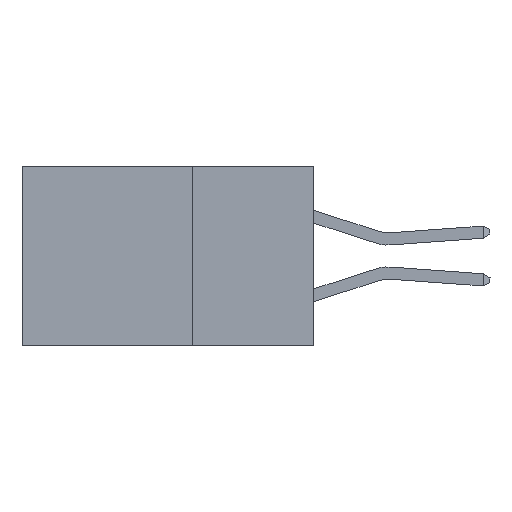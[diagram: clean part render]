
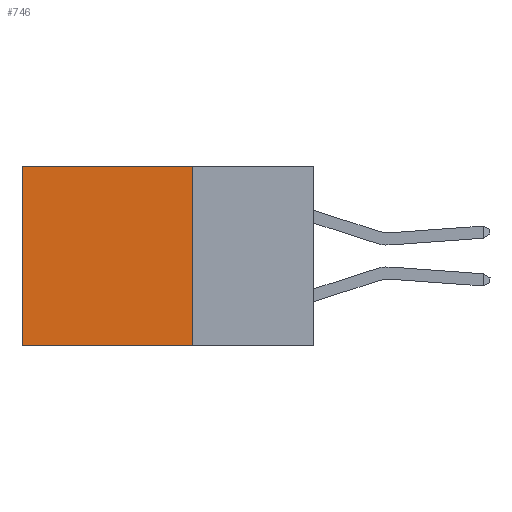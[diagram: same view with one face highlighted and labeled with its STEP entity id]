
A CAD part, left-side view. The second image highlights one B-rep face of the part: STEP entity #746.
In plain terms, the highlighted planar face has unit normal (-1, 0, 0).
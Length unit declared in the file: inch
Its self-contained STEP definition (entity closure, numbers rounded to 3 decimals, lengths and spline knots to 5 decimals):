
#235 = CARTESIAN_POINT ( 'NONE',  ( 0.2875, 0.25, -0.37 ) ) ;
#746 = ADVANCED_FACE ( 'NONE', ( #23379 ), #26019, .F. ) ;
#1162 = CARTESIAN_POINT ( 'NONE',  ( 0.2875, 0.25, 0. ) ) ;
#1590 = VERTEX_POINT ( 'NONE', #28238 ) ;
#2686 = DIRECTION ( 'NONE',  ( 0., 0., -1. ) ) ;
#2745 = CARTESIAN_POINT ( 'NONE',  ( 0.2875, 0.25, 0. ) ) ;
#2875 = DIRECTION ( 'NONE',  ( 0., 1., 0. ) ) ;
#3128 = CARTESIAN_POINT ( 'NONE',  ( 0.2875, 0.6, -0.37 ) ) ;
#3376 = DIRECTION ( 'NONE',  ( 1., 0., 0. ) ) ;
#5682 = EDGE_CURVE ( 'NONE', #7525, #10924, #10752, .T. ) ;
#6465 = EDGE_CURVE ( 'NONE', #19466, #7525, #8320, .T. ) ;
#6934 = ORIENTED_EDGE ( 'NONE', *, *, #10051, .F. ) ;
#7165 = LINE ( 'NONE', #235, #14205 ) ;
#7525 = VERTEX_POINT ( 'NONE', #18082 ) ;
#8046 = CARTESIAN_POINT ( 'NONE',  ( 0.2875, 0.25, 0. ) ) ;
#8320 = LINE ( 'NONE', #2745, #20959 ) ;
#9557 = AXIS2_PLACEMENT_3D ( 'NONE', #8046, #3376, #23867 ) ;
#9558 = DIRECTION ( 'NONE',  ( 0., 1., 0. ) ) ;
#10051 = EDGE_CURVE ( 'NONE', #19466, #1590, #17558, .T. ) ;
#10064 = ORIENTED_EDGE ( 'NONE', *, *, #6465, .T. ) ;
#10752 = LINE ( 'NONE', #16939, #27661 ) ;
#10924 = VERTEX_POINT ( 'NONE', #3128 ) ;
#14205 = VECTOR ( 'NONE', #2875, 39.37008 ) ;
#16939 = CARTESIAN_POINT ( 'NONE',  ( 0.2875, 0.6, 0. ) ) ;
#17558 = LINE ( 'NONE', #20416, #21056 ) ;
#18082 = CARTESIAN_POINT ( 'NONE',  ( 0.2875, 0.6, 0. ) ) ;
#19466 = VERTEX_POINT ( 'NONE', #1162 ) ;
#19820 = EDGE_CURVE ( 'NONE', #1590, #10924, #7165, .T. ) ;
#20298 = ORIENTED_EDGE ( 'NONE', *, *, #19820, .F. ) ;
#20416 = CARTESIAN_POINT ( 'NONE',  ( 0.2875, 0.25, 0. ) ) ;
#20959 = VECTOR ( 'NONE', #9558, 39.37008 ) ;
#21056 = VECTOR ( 'NONE', #2686, 39.37008 ) ;
#21446 = DIRECTION ( 'NONE',  ( 0., 0., -1. ) ) ;
#23379 = FACE_OUTER_BOUND ( 'NONE', #28223, .T. ) ;
#23867 = DIRECTION ( 'NONE',  ( 0., 0., -1. ) ) ;
#26019 = PLANE ( 'NONE',  #9557 ) ;
#27283 = ORIENTED_EDGE ( 'NONE', *, *, #5682, .T. ) ;
#27661 = VECTOR ( 'NONE', #21446, 39.37008 ) ;
#28223 = EDGE_LOOP ( 'NONE', ( #27283, #20298, #6934, #10064 ) ) ;
#28238 = CARTESIAN_POINT ( 'NONE',  ( 0.2875, 0.25, -0.37 ) ) ;
